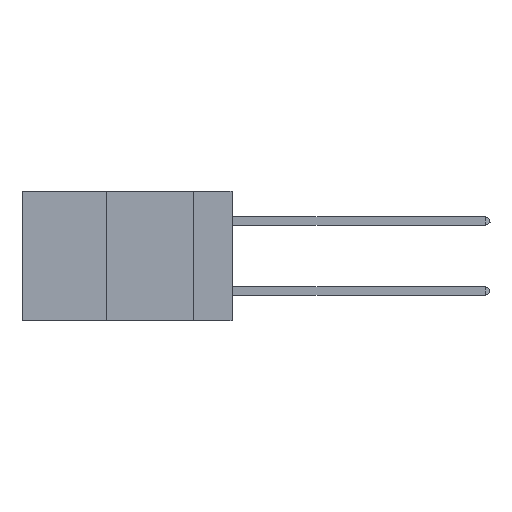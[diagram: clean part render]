
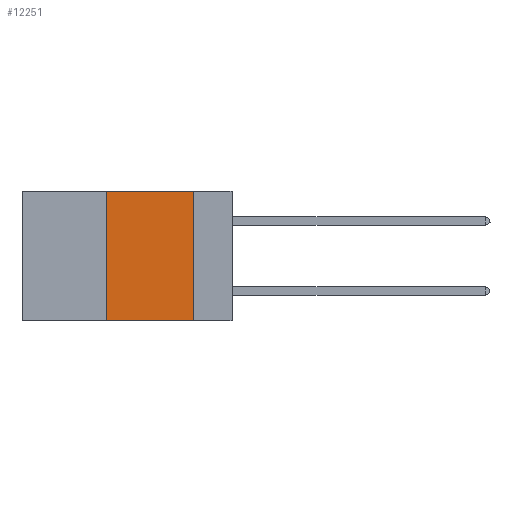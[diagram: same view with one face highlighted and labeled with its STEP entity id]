
A CAD part, left-side view. The second image highlights one B-rep face of the part: STEP entity #12251.
In plain terms, the highlighted planar face has unit normal (-1, 0, 0).
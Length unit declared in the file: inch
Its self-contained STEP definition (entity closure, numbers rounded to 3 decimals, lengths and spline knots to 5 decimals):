
#52 = FACE_OUTER_BOUND ( 'NONE', #4988, .T. ) ;
#432 = ORIENTED_EDGE ( 'NONE', *, *, #6051, .F. ) ;
#835 = DIRECTION ( 'NONE',  ( 0., -1., 0. ) ) ;
#881 = VERTEX_POINT ( 'NONE', #8464 ) ;
#918 = CARTESIAN_POINT ( 'NONE',  ( 0., 0.6, -0.37 ) ) ;
#1018 = LINE ( 'NONE', #13728, #7047 ) ;
#3331 = DIRECTION ( 'NONE',  ( 0., 0., -1. ) ) ;
#3456 = LINE ( 'NONE', #918, #8663 ) ;
#3671 = LINE ( 'NONE', #9419, #4397 ) ;
#4397 = VECTOR ( 'NONE', #7736, 39.37008 ) ;
#4696 = ORIENTED_EDGE ( 'NONE', *, *, #11409, .T. ) ;
#4870 = DIRECTION ( 'NONE',  ( 0., -1., 0. ) ) ;
#4988 = EDGE_LOOP ( 'NONE', ( #432, #12414, #9800, #4696 ) ) ;
#5761 = CARTESIAN_POINT ( 'NONE',  ( 0., 0.11, 0. ) ) ;
#5905 = CARTESIAN_POINT ( 'NONE',  ( 0., 0.36, 0. ) ) ;
#5918 = VERTEX_POINT ( 'NONE', #5761 ) ;
#6051 = EDGE_CURVE ( 'NONE', #5918, #17961, #12001, .T. ) ;
#6571 = EDGE_CURVE ( 'NONE', #11193, #5918, #1018, .T. ) ;
#7047 = VECTOR ( 'NONE', #835, 39.37008 ) ;
#7736 = DIRECTION ( 'NONE',  ( 0., 0., 1. ) ) ;
#8464 = CARTESIAN_POINT ( 'NONE',  ( 0., 0.36, -0.37 ) ) ;
#8606 = DIRECTION ( 'NONE',  ( 1., 0., 0. ) ) ;
#8663 = VECTOR ( 'NONE', #4870, 39.37008 ) ;
#9419 = CARTESIAN_POINT ( 'NONE',  ( 0., 0.36, 0. ) ) ;
#9592 = DIRECTION ( 'NONE',  ( 0., 0., -1. ) ) ;
#9597 = EDGE_CURVE ( 'NONE', #881, #11193, #3671, .T. ) ;
#9800 = ORIENTED_EDGE ( 'NONE', *, *, #9597, .F. ) ;
#10500 = CARTESIAN_POINT ( 'NONE',  ( 0., 0.11, 0. ) ) ;
#11193 = VERTEX_POINT ( 'NONE', #5905 ) ;
#11409 = EDGE_CURVE ( 'NONE', #881, #17961, #3456, .T. ) ;
#11437 = PLANE ( 'NONE',  #16520 ) ;
#12001 = LINE ( 'NONE', #10500, #15484 ) ;
#12251 = ADVANCED_FACE ( 'NONE', ( #52 ), #11437, .F. ) ;
#12263 = CARTESIAN_POINT ( 'NONE',  ( 0., 0.11, -0.37 ) ) ;
#12414 = ORIENTED_EDGE ( 'NONE', *, *, #6571, .F. ) ;
#13728 = CARTESIAN_POINT ( 'NONE',  ( 0., 0.6, 0. ) ) ;
#15484 = VECTOR ( 'NONE', #9592, 39.37008 ) ;
#16520 = AXIS2_PLACEMENT_3D ( 'NONE', #17182, #8606, #3331 ) ;
#17182 = CARTESIAN_POINT ( 'NONE',  ( 0., 0.6, 0. ) ) ;
#17961 = VERTEX_POINT ( 'NONE', #12263 ) ;
